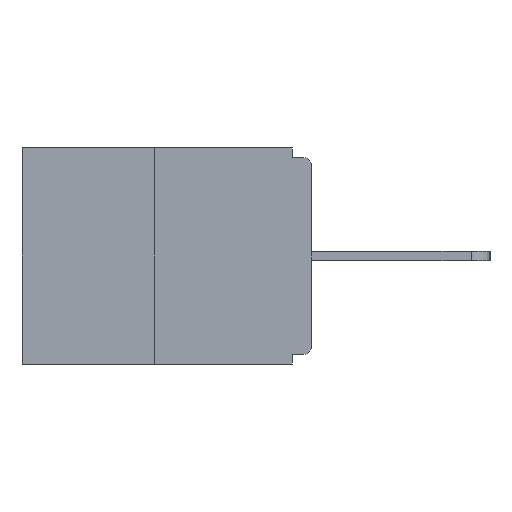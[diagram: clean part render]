
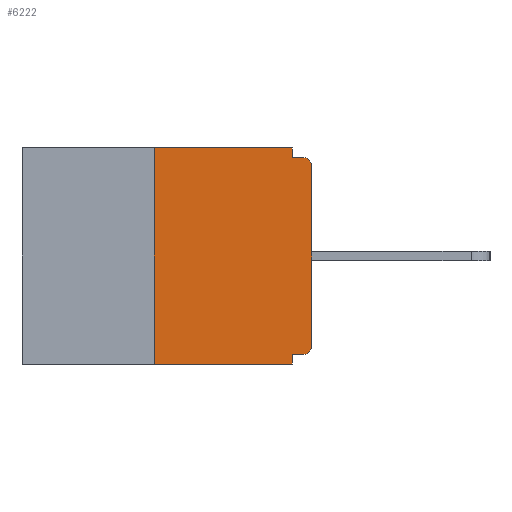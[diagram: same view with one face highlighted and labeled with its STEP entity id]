
A CAD part, left-side view. The second image highlights one B-rep face of the part: STEP entity #6222.
In plain terms, the highlighted planar face has unit normal (-1, 0, 0).
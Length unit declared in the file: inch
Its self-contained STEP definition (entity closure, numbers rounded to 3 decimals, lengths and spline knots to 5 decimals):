
#491 = CIRCLE ( 'NONE', #3937, 0.015 ) ;
#511 = CARTESIAN_POINT ( 'NONE',  ( 0., 0., -0.328 ) ) ;
#630 = ORIENTED_EDGE ( 'NONE', *, *, #9304, .T. ) ;
#670 = VECTOR ( 'NONE', #4087, 39.37008 ) ;
#777 = CARTESIAN_POINT ( 'NONE',  ( 0., 0.031, -0.343 ) ) ;
#917 = CARTESIAN_POINT ( 'NONE',  ( 0., 0., -0.03 ) ) ;
#922 = VERTEX_POINT ( 'NONE', #917 ) ;
#978 = AXIS2_PLACEMENT_3D ( 'NONE', #4934, #9717, #1973 ) ;
#1077 = EDGE_CURVE ( 'NONE', #12332, #9859, #2875, .T. ) ;
#1126 = CARTESIAN_POINT ( 'NONE',  ( 0., 0.031, 0. ) ) ;
#1649 = VERTEX_POINT ( 'NONE', #8294 ) ;
#1798 = CARTESIAN_POINT ( 'NONE',  ( 0., 0.46, -0.343 ) ) ;
#1830 = ORIENTED_EDGE ( 'NONE', *, *, #6064, .F. ) ;
#1973 = DIRECTION ( 'NONE',  ( 0., 0., -1. ) ) ;
#2135 = DIRECTION ( 'NONE',  ( 0., 0., -1. ) ) ;
#2234 = CARTESIAN_POINT ( 'NONE',  ( 0., 0.46, 0. ) ) ;
#2249 = ORIENTED_EDGE ( 'NONE', *, *, #11120, .T. ) ;
#2404 = CARTESIAN_POINT ( 'NONE',  ( 0., 0.46, 0. ) ) ;
#2495 = VERTEX_POINT ( 'NONE', #11675 ) ;
#2834 = VECTOR ( 'NONE', #8940, 39.37008 ) ;
#2875 = LINE ( 'NONE', #7003, #2834 ) ;
#3010 = FACE_OUTER_BOUND ( 'NONE', #5244, .T. ) ;
#3348 = VERTEX_POINT ( 'NONE', #4864 ) ;
#3476 = VECTOR ( 'NONE', #3994, 39.37008 ) ;
#3533 = ORIENTED_EDGE ( 'NONE', *, *, #6782, .F. ) ;
#3619 = LINE ( 'NONE', #4577, #8278 ) ;
#3937 = AXIS2_PLACEMENT_3D ( 'NONE', #6885, #9775, #8838 ) ;
#3994 = DIRECTION ( 'NONE',  ( 0., 0., 1. ) ) ;
#4072 = LINE ( 'NONE', #1126, #4254 ) ;
#4087 = DIRECTION ( 'NONE',  ( 0., -1., 0. ) ) ;
#4166 = CARTESIAN_POINT ( 'NONE',  ( 0., 0.031, -0.328 ) ) ;
#4193 = ORIENTED_EDGE ( 'NONE', *, *, #9979, .F. ) ;
#4254 = VECTOR ( 'NONE', #2135, 39.37008 ) ;
#4577 = CARTESIAN_POINT ( 'NONE',  ( 0., 0.25, 0. ) ) ;
#4622 = EDGE_CURVE ( 'NONE', #8268, #9276, #3619, .T. ) ;
#4864 = CARTESIAN_POINT ( 'NONE',  ( 0., 0.031, -0.343 ) ) ;
#4934 = CARTESIAN_POINT ( 'NONE',  ( 0., 0.015, -0.313 ) ) ;
#5244 = EDGE_LOOP ( 'NONE', ( #4193, #7359, #630, #1830, #3533, #8698, #10907, #2249, #8348, #7697 ) ) ;
#5440 = CARTESIAN_POINT ( 'NONE',  ( 0., 0.031, 0. ) ) ;
#5720 = VECTOR ( 'NONE', #12429, 39.37008 ) ;
#5835 = EDGE_CURVE ( 'NONE', #6734, #12332, #4072, .T. ) ;
#5915 = AXIS2_PLACEMENT_3D ( 'NONE', #2234, #11744, #6852 ) ;
#6064 = EDGE_CURVE ( 'NONE', #6607, #3348, #6606, .T. ) ;
#6079 = PLANE ( 'NONE',  #5915 ) ;
#6222 = ADVANCED_FACE ( 'NONE', ( #3010 ), #6079, .F. ) ;
#6386 = LINE ( 'NONE', #511, #7352 ) ;
#6606 = LINE ( 'NONE', #777, #6698 ) ;
#6607 = VERTEX_POINT ( 'NONE', #4166 ) ;
#6698 = VECTOR ( 'NONE', #8500, 39.37008 ) ;
#6734 = VERTEX_POINT ( 'NONE', #5440 ) ;
#6782 = EDGE_CURVE ( 'NONE', #1649, #6607, #6386, .T. ) ;
#6825 = CARTESIAN_POINT ( 'NONE',  ( 0., 0.015, -0.015 ) ) ;
#6829 = CARTESIAN_POINT ( 'NONE',  ( 0., 0.25, -0.343 ) ) ;
#6852 = DIRECTION ( 'NONE',  ( 0., 0., -1. ) ) ;
#6885 = CARTESIAN_POINT ( 'NONE',  ( 0., 0.015, -0.03 ) ) ;
#6897 = LINE ( 'NONE', #10552, #3476 ) ;
#7003 = CARTESIAN_POINT ( 'NONE',  ( 0., 0., -0.015 ) ) ;
#7025 = EDGE_CURVE ( 'NONE', #1649, #2495, #8234, .T. ) ;
#7352 = VECTOR ( 'NONE', #8282, 39.37008 ) ;
#7359 = ORIENTED_EDGE ( 'NONE', *, *, #4622, .F. ) ;
#7613 = CARTESIAN_POINT ( 'NONE',  ( 0., 0.031, -0.015 ) ) ;
#7697 = ORIENTED_EDGE ( 'NONE', *, *, #5835, .F. ) ;
#8234 = CIRCLE ( 'NONE', #978, 0.015 ) ;
#8268 = VERTEX_POINT ( 'NONE', #6829 ) ;
#8278 = VECTOR ( 'NONE', #10307, 39.37008 ) ;
#8282 = DIRECTION ( 'NONE',  ( 0., 1., 0. ) ) ;
#8294 = CARTESIAN_POINT ( 'NONE',  ( 0., 0.015, -0.328 ) ) ;
#8348 = ORIENTED_EDGE ( 'NONE', *, *, #1077, .F. ) ;
#8500 = DIRECTION ( 'NONE',  ( 0., 0., -1. ) ) ;
#8698 = ORIENTED_EDGE ( 'NONE', *, *, #7025, .T. ) ;
#8838 = DIRECTION ( 'NONE',  ( 0., 0., -1. ) ) ;
#8940 = DIRECTION ( 'NONE',  ( 0., -1., 0. ) ) ;
#9129 = LINE ( 'NONE', #2404, #670 ) ;
#9276 = VERTEX_POINT ( 'NONE', #11496 ) ;
#9304 = EDGE_CURVE ( 'NONE', #8268, #3348, #10414, .T. ) ;
#9450 = EDGE_CURVE ( 'NONE', #2495, #922, #6897, .T. ) ;
#9717 = DIRECTION ( 'NONE',  ( -1., 0., 0. ) ) ;
#9775 = DIRECTION ( 'NONE',  ( -1., 0., 0. ) ) ;
#9859 = VERTEX_POINT ( 'NONE', #6825 ) ;
#9979 = EDGE_CURVE ( 'NONE', #9276, #6734, #9129, .T. ) ;
#10307 = DIRECTION ( 'NONE',  ( 0., 0., 1. ) ) ;
#10414 = LINE ( 'NONE', #1798, #5720 ) ;
#10552 = CARTESIAN_POINT ( 'NONE',  ( 0., 0., 0. ) ) ;
#10907 = ORIENTED_EDGE ( 'NONE', *, *, #9450, .T. ) ;
#11120 = EDGE_CURVE ( 'NONE', #922, #9859, #491, .T. ) ;
#11496 = CARTESIAN_POINT ( 'NONE',  ( 0., 0.25, 0. ) ) ;
#11675 = CARTESIAN_POINT ( 'NONE',  ( 0., 0., -0.313 ) ) ;
#11744 = DIRECTION ( 'NONE',  ( 1., 0., 0. ) ) ;
#12332 = VERTEX_POINT ( 'NONE', #7613 ) ;
#12429 = DIRECTION ( 'NONE',  ( 0., -1., 0. ) ) ;
